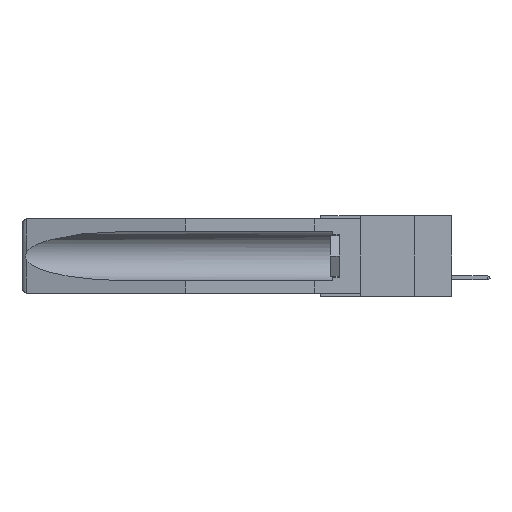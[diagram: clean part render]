
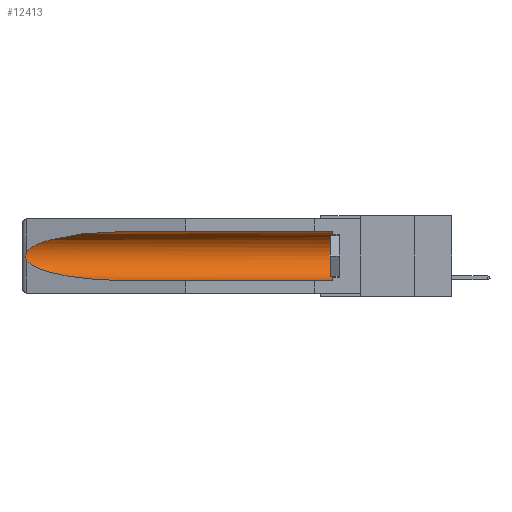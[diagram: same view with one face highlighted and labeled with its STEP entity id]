
A CAD part, left-side view. The second image highlights one B-rep face of the part: STEP entity #12413.
In plain terms, the highlighted cylindrical face has radius 2.857 mm (diameter 5.715 mm), a partial arc.
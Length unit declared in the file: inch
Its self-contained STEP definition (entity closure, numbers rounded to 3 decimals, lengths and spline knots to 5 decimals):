
#293 = CARTESIAN_POINT ( 'NONE',  ( 0.26537, 1.52718, -0.14972 ) ) ;
#568 = CARTESIAN_POINT ( 'NONE',  ( 0.155, 0.126, -0.059 ) ) ;
#733 = VECTOR ( 'NONE', #12585, 39.37008 ) ;
#1106 = DIRECTION ( 'NONE',  ( 0., 0., 1. ) ) ;
#1575 = CARTESIAN_POINT ( 'NONE',  ( 0.155, -0.30754, -0.059 ) ) ;
#1652 = CARTESIAN_POINT ( 'NONE',  ( 0.26597, 1.52961, -0.15275 ) ) ;
#2907 = CIRCLE ( 'NONE', #13233, 0.1125 ) ;
#3776 = DIRECTION ( 'NONE',  ( 0., 1., 0. ) ) ;
#4863 = CARTESIAN_POINT ( 'NONE',  ( 0.155, 1.07973, -0.284 ) ) ;
#5724 = CARTESIAN_POINT ( 'NONE',  ( 0.155, 0.126, -0.1715 ) ) ;
#6604 = CARTESIAN_POINT ( 'NONE',  ( 0.26537, 1.52718, -0.14972 ) ) ;
#7657 = CARTESIAN_POINT ( 'NONE',  ( 0.155, -0.30754, -0.284 ) ) ;
#7866 = EDGE_CURVE ( 'NONE', #22146, #9770, #22315, .T. ) ;
#8085 = CARTESIAN_POINT ( 'NONE',  ( 0.2673, 1.53269, -0.17917 ) ) ;
#8226 = EDGE_LOOP ( 'NONE', ( #23245, #18082, #26035, #25020, #22136, #15450 ) ) ;
#9568 = AXIS2_PLACEMENT_3D ( 'NONE', #25611, #3776, #10535 ) ;
#9770 = VERTEX_POINT ( 'NONE', #22905 ) ;
#10260 = CARTESIAN_POINT ( 'NONE',  ( 0.26597, 1.5296, -0.19026 ) ) ;
#10322 = VERTEX_POINT ( 'NONE', #24188 ) ;
#10535 = DIRECTION ( 'NONE',  ( 0., 0., 1. ) ) ;
#10882 = CARTESIAN_POINT ( 'NONE',  ( 0.155, 1.07973, -0.284 ) ) ;
#11297 = CARTESIAN_POINT ( 'NONE',  ( 0.155, 1.07973, -0.059 ) ) ;
#11520 = VERTEX_POINT ( 'NONE', #10882 ) ;
#11803 = EDGE_CURVE ( 'NONE', #17467, #22146, #2907, .T. ) ;
#12190 = CARTESIAN_POINT ( 'NONE',  ( 0.2675, 1.53308, -0.17534 ) ) ;
#12385 = CARTESIAN_POINT ( 'NONE',  ( 0.26537, 1.52718, -0.14972 ) ) ;
#12413 = ADVANCED_FACE ( 'NONE', ( #13497 ), #15887, .F. ) ;
#12568 = CARTESIAN_POINT ( 'NONE',  ( 0.26654, 1.53092, -0.15636 ) ) ;
#12585 = DIRECTION ( 'NONE',  ( 0., 1., 0. ) ) ;
#13233 = AXIS2_PLACEMENT_3D ( 'NONE', #5724, #27611, #1106 ) ;
#13497 = FACE_OUTER_BOUND ( 'NONE', #8226, .T. ) ;
#14165 = EDGE_CURVE ( 'NONE', #17467, #11520, #26987, .T. ) ;
#14808 = CARTESIAN_POINT ( 'NONE',  ( 0.26655, 1.53094, -0.18657 ) ) ;
#15161 = EDGE_CURVE ( 'NONE', #10322, #11520, #24402, .T. ) ;
#15298 = CARTESIAN_POINT ( 'NONE',  ( 0.26537, 1.52718, -0.19328 ) ) ;
#15450 = ORIENTED_EDGE ( 'NONE', *, *, #7866, .T. ) ;
#15887 = CYLINDRICAL_SURFACE ( 'NONE', #9568, 0.1125 ) ;
#17467 = VERTEX_POINT ( 'NONE', #17662 ) ;
#17662 = CARTESIAN_POINT ( 'NONE',  ( 0.155, 0.126, -0.284 ) ) ;
#17938 = CARTESIAN_POINT ( 'NONE',  ( 0.21114, 1.30732, -0.059 ) ) ;
#18034 = CARTESIAN_POINT ( 'NONE',  ( 0.25451, 1.48313, -0.09465 ) ) ;
#18082 = ORIENTED_EDGE ( 'NONE', *, *, #19021, .T. ) ;
#18663 = VERTEX_POINT ( 'NONE', #6604 ) ;
#19021 = EDGE_CURVE ( 'NONE', #18663, #10322, #19824, .T. ) ;
#19711 = CARTESIAN_POINT ( 'NONE',  ( 0.25451, 1.48313, -0.24835 ) ) ;
#19824 = B_SPLINE_CURVE_WITH_KNOTS ( 'NONE', 3,
 ( #12385, #1652, #12568, #21194, #25328, #12190, #8085, #14808, #10260, #25609 ),
 .UNSPECIFIED., .F., .F.,
 ( 4, 2, 2, 2, 4 ),
 ( 0., 0.00029, 0.00058, 0.00087, 0.00117 ),
 .UNSPECIFIED. ) ;
#20689 = DIRECTION ( 'NONE',  ( 0., 1., 0. ) ) ;
#21175 = VECTOR ( 'NONE', #20689, 39.37008 ) ;
#21194 = CARTESIAN_POINT ( 'NONE',  ( 0.2673, 1.5327, -0.16383 ) ) ;
#21575 = EDGE_CURVE ( 'NONE', #9770, #18663, #24032, .T. ) ;
#22136 = ORIENTED_EDGE ( 'NONE', *, *, #11803, .T. ) ;
#22146 = VERTEX_POINT ( 'NONE', #568 ) ;
#22315 = LINE ( 'NONE', #1575, #733 ) ;
#22368 = CARTESIAN_POINT ( 'NONE',  ( 0.21114, 1.30732, -0.284 ) ) ;
#22905 = CARTESIAN_POINT ( 'NONE',  ( 0.155, 1.07973, -0.059 ) ) ;
#23245 = ORIENTED_EDGE ( 'NONE', *, *, #21575, .T. ) ;
#24032 =( BOUNDED_CURVE ( )  B_SPLINE_CURVE ( 3, ( #11297, #17938, #18034, #293 ),
 .UNSPECIFIED., .F., .F. ) 
 B_SPLINE_CURVE_WITH_KNOTS ( ( 4, 4 ),
 ( 4.71239, 6.08839 ),
 .UNSPECIFIED. ) 
 CURVE ( )  GEOMETRIC_REPRESENTATION_ITEM ( )  RATIONAL_B_SPLINE_CURVE ( ( 1., 0.848, 0.848, 1. ) ) 
 REPRESENTATION_ITEM ( '' )  );
#24188 = CARTESIAN_POINT ( 'NONE',  ( 0.26537, 1.52718, -0.19328 ) ) ;
#24402 =( BOUNDED_CURVE ( )  B_SPLINE_CURVE ( 3, ( #15298, #19711, #22368, #4863 ),
 .UNSPECIFIED., .F., .F. ) 
 B_SPLINE_CURVE_WITH_KNOTS ( ( 4, 4 ),
 ( 0.1948, 1.5708 ),
 .UNSPECIFIED. ) 
 CURVE ( )  GEOMETRIC_REPRESENTATION_ITEM ( )  RATIONAL_B_SPLINE_CURVE ( ( 1., 0.848, 0.848, 1. ) ) 
 REPRESENTATION_ITEM ( '' )  );
#25020 = ORIENTED_EDGE ( 'NONE', *, *, #14165, .F. ) ;
#25328 = CARTESIAN_POINT ( 'NONE',  ( 0.2675, 1.53308, -0.16763 ) ) ;
#25609 = CARTESIAN_POINT ( 'NONE',  ( 0.26537, 1.52718, -0.19328 ) ) ;
#25611 = CARTESIAN_POINT ( 'NONE',  ( 0.155, -0.30754, -0.1715 ) ) ;
#26035 = ORIENTED_EDGE ( 'NONE', *, *, #15161, .T. ) ;
#26987 = LINE ( 'NONE', #7657, #21175 ) ;
#27611 = DIRECTION ( 'NONE',  ( 0., -1., 0. ) ) ;
